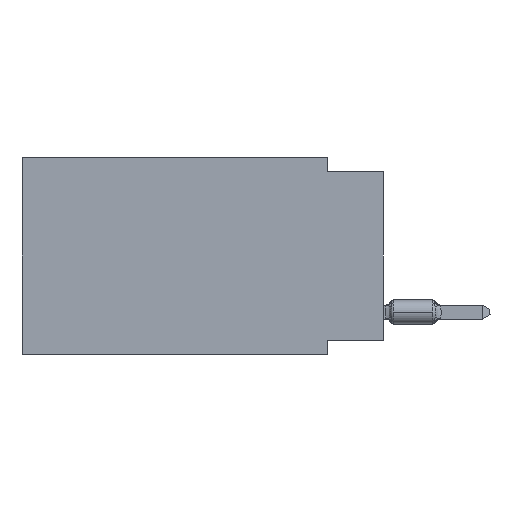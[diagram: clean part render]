
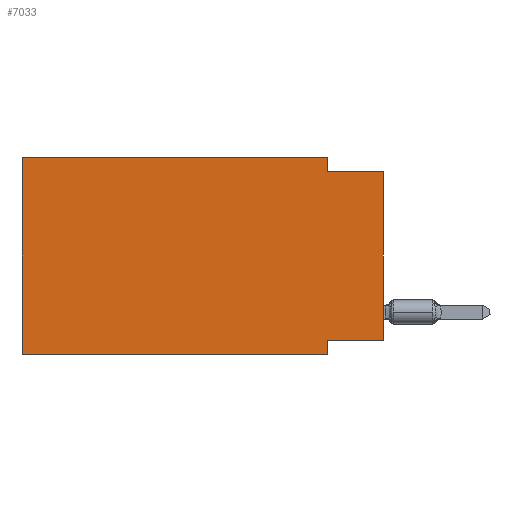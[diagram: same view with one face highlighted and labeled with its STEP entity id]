
A CAD part, left-side view. The second image highlights one B-rep face of the part: STEP entity #7033.
In plain terms, the highlighted planar face has unit normal (-1, 0, 0).
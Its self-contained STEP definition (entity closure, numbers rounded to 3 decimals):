
#1307 = ORIENTED_EDGE ( 'NONE', *, *, #48061, .T. ) ;
#2235 = CARTESIAN_POINT ( 'NONE',  ( 0., 2.54, -8.89 ) ) ;
#2619 = DIRECTION ( 'NONE',  ( 1., 0., 0. ) ) ;
#2910 = VERTEX_POINT ( 'NONE', #2235 ) ;
#2941 = ORIENTED_EDGE ( 'NONE', *, *, #6042, .F. ) ;
#3636 = CARTESIAN_POINT ( 'NONE',  ( 0., 2.54, -0.635 ) ) ;
#3677 = CARTESIAN_POINT ( 'NONE',  ( 0., 0., -0.635 ) ) ;
#3826 = VERTEX_POINT ( 'NONE', #3636 ) ;
#4112 = LINE ( 'NONE', #29408, #11865 ) ;
#6042 = EDGE_CURVE ( 'NONE', #28395, #35475, #14740, .T. ) ;
#6634 = VERTEX_POINT ( 'NONE', #52219 ) ;
#6654 = CARTESIAN_POINT ( 'NONE',  ( 0., 2.54, -8.255 ) ) ;
#6770 = DIRECTION ( 'NONE',  ( 0., 0., -1. ) ) ;
#7033 = ADVANCED_FACE ( 'NONE', ( #11156 ), #44201, .F. ) ;
#7111 = CARTESIAN_POINT ( 'NONE',  ( 0., 2.54, -8.89 ) ) ;
#7388 = VERTEX_POINT ( 'NONE', #45761 ) ;
#7875 = CARTESIAN_POINT ( 'NONE',  ( 0., 0., -8.255 ) ) ;
#8788 = EDGE_CURVE ( 'NONE', #6634, #42366, #36145, .T. ) ;
#10628 = ORIENTED_EDGE ( 'NONE', *, *, #38638, .F. ) ;
#11156 = FACE_OUTER_BOUND ( 'NONE', #43998, .T. ) ;
#11865 = VECTOR ( 'NONE', #17172, 1000. ) ;
#11964 = EDGE_CURVE ( 'NONE', #3826, #7388, #51913, .T. ) ;
#13490 = CARTESIAN_POINT ( 'NONE',  ( 0., 16.383, 0. ) ) ;
#14740 = LINE ( 'NONE', #17979, #37041 ) ;
#15424 = DIRECTION ( 'NONE',  ( 0., -1., 0. ) ) ;
#17172 = DIRECTION ( 'NONE',  ( 0., -1., 0. ) ) ;
#17338 = VERTEX_POINT ( 'NONE', #41791 ) ;
#17979 = CARTESIAN_POINT ( 'NONE',  ( 0., 16.383, 0. ) ) ;
#18638 = DIRECTION ( 'NONE',  ( 0., 0., -1. ) ) ;
#19132 = ORIENTED_EDGE ( 'NONE', *, *, #44792, .F. ) ;
#21789 = VECTOR ( 'NONE', #32146, 1000. ) ;
#25017 = LINE ( 'NONE', #41277, #30438 ) ;
#25878 = AXIS2_PLACEMENT_3D ( 'NONE', #31668, #2619, #18638 ) ;
#26145 = CARTESIAN_POINT ( 'NONE',  ( 0., 16.383, -8.89 ) ) ;
#27572 = LINE ( 'NONE', #27849, #52574 ) ;
#27668 = DIRECTION ( 'NONE',  ( 0., 0., -1. ) ) ;
#27849 = CARTESIAN_POINT ( 'NONE',  ( 0., 2.54, 0. ) ) ;
#28395 = VERTEX_POINT ( 'NONE', #26145 ) ;
#28529 = ORIENTED_EDGE ( 'NONE', *, *, #48324, .T. ) ;
#29035 = DIRECTION ( 'NONE',  ( 0., 0., 1. ) ) ;
#29408 = CARTESIAN_POINT ( 'NONE',  ( 0., 16.383, 0. ) ) ;
#30438 = VECTOR ( 'NONE', #29035, 1000. ) ;
#31391 = LINE ( 'NONE', #7111, #52268 ) ;
#31668 = CARTESIAN_POINT ( 'NONE',  ( 0., 16.383, 0. ) ) ;
#32146 = DIRECTION ( 'NONE',  ( 0., 1., 0. ) ) ;
#33796 = ORIENTED_EDGE ( 'NONE', *, *, #39969, .F. ) ;
#34824 = LINE ( 'NONE', #51064, #51659 ) ;
#35475 = VERTEX_POINT ( 'NONE', #13490 ) ;
#36145 = LINE ( 'NONE', #7875, #21789 ) ;
#36788 = VECTOR ( 'NONE', #15424, 1000. ) ;
#37041 = VECTOR ( 'NONE', #50453, 1000. ) ;
#38638 = EDGE_CURVE ( 'NONE', #17338, #3826, #27572, .T. ) ;
#39969 = EDGE_CURVE ( 'NONE', #35475, #17338, #4112, .T. ) ;
#41277 = CARTESIAN_POINT ( 'NONE',  ( 0., 0., 0. ) ) ;
#41791 = CARTESIAN_POINT ( 'NONE',  ( 0., 2.54, 0. ) ) ;
#42366 = VERTEX_POINT ( 'NONE', #6654 ) ;
#43998 = EDGE_LOOP ( 'NONE', ( #28529, #45204, #10628, #33796, #2941, #1307, #19132, #50415 ) ) ;
#44201 = PLANE ( 'NONE',  #25878 ) ;
#44792 = EDGE_CURVE ( 'NONE', #42366, #2910, #31391, .T. ) ;
#45204 = ORIENTED_EDGE ( 'NONE', *, *, #11964, .F. ) ;
#45761 = CARTESIAN_POINT ( 'NONE',  ( 0., 0., -0.635 ) ) ;
#47070 = DIRECTION ( 'NONE',  ( 0., -1., 0. ) ) ;
#48061 = EDGE_CURVE ( 'NONE', #28395, #2910, #34824, .T. ) ;
#48324 = EDGE_CURVE ( 'NONE', #6634, #7388, #25017, .T. ) ;
#50415 = ORIENTED_EDGE ( 'NONE', *, *, #8788, .F. ) ;
#50453 = DIRECTION ( 'NONE',  ( 0., 0., 1. ) ) ;
#51064 = CARTESIAN_POINT ( 'NONE',  ( 0., 16.383, -8.89 ) ) ;
#51659 = VECTOR ( 'NONE', #47070, 1000. ) ;
#51913 = LINE ( 'NONE', #3677, #36788 ) ;
#52219 = CARTESIAN_POINT ( 'NONE',  ( 0., 0., -8.255 ) ) ;
#52268 = VECTOR ( 'NONE', #27668, 1000. ) ;
#52574 = VECTOR ( 'NONE', #6770, 1000. ) ;
